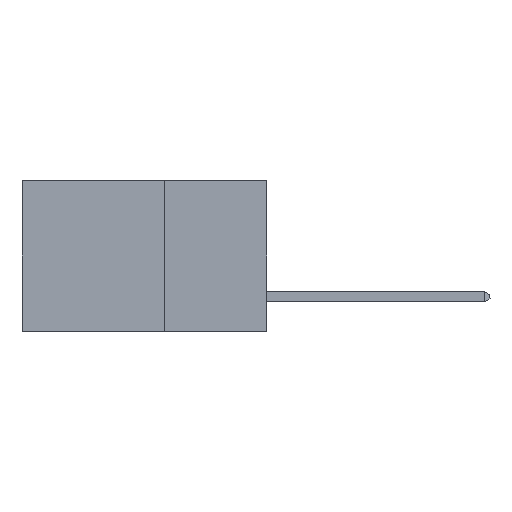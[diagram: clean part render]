
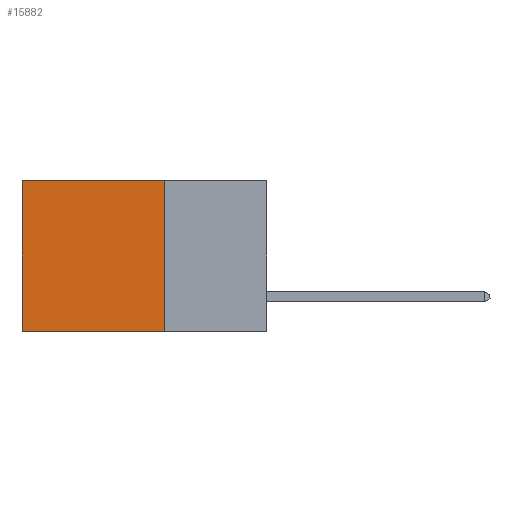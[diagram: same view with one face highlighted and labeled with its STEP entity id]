
A CAD part, left-side view. The second image highlights one B-rep face of the part: STEP entity #15882.
In plain terms, the highlighted planar face has unit normal (-1, 0, 0).
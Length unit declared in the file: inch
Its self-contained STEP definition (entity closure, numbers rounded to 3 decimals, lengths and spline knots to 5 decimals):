
#60 = CARTESIAN_POINT ( 'NONE',  ( 0.2875, 0.25, -0.37 ) ) ;
#1473 = LINE ( 'NONE', #2595, #8041 ) ;
#2060 = ORIENTED_EDGE ( 'NONE', *, *, #10140, .T. ) ;
#2313 = CARTESIAN_POINT ( 'NONE',  ( 0.2875, 0.25, 0. ) ) ;
#2595 = CARTESIAN_POINT ( 'NONE',  ( 0.2875, 0.6, 0. ) ) ;
#3277 = VERTEX_POINT ( 'NONE', #14177 ) ;
#4044 = DIRECTION ( 'NONE',  ( 0., 0., -1. ) ) ;
#4295 = PLANE ( 'NONE',  #15680 ) ;
#4554 = VECTOR ( 'NONE', #10521, 39.37008 ) ;
#4685 = VERTEX_POINT ( 'NONE', #15524 ) ;
#4790 = ORIENTED_EDGE ( 'NONE', *, *, #6001, .T. ) ;
#5188 = CARTESIAN_POINT ( 'NONE',  ( 0.2875, 0.25, -0.37 ) ) ;
#5407 = LINE ( 'NONE', #2313, #4554 ) ;
#6001 = EDGE_CURVE ( 'NONE', #12307, #3277, #5407, .T. ) ;
#6719 = FACE_OUTER_BOUND ( 'NONE', #9423, .T. ) ;
#7062 = DIRECTION ( 'NONE',  ( 0., 0., -1. ) ) ;
#7885 = ORIENTED_EDGE ( 'NONE', *, *, #8242, .F. ) ;
#7898 = EDGE_CURVE ( 'NONE', #12307, #12580, #13830, .T. ) ;
#8041 = VECTOR ( 'NONE', #4044, 39.37008 ) ;
#8242 = EDGE_CURVE ( 'NONE', #12580, #4685, #14992, .T. ) ;
#8834 = CARTESIAN_POINT ( 'NONE',  ( 0.2875, 0.25, 0. ) ) ;
#9423 = EDGE_LOOP ( 'NONE', ( #2060, #7885, #16205, #4790 ) ) ;
#10140 = EDGE_CURVE ( 'NONE', #3277, #4685, #1473, .T. ) ;
#10419 = VECTOR ( 'NONE', #10438, 39.37008 ) ;
#10438 = DIRECTION ( 'NONE',  ( 0., 0., -1. ) ) ;
#10521 = DIRECTION ( 'NONE',  ( 0., 1., 0. ) ) ;
#11008 = CARTESIAN_POINT ( 'NONE',  ( 0.2875, 0.25, 0. ) ) ;
#11138 = DIRECTION ( 'NONE',  ( 0., 1., 0. ) ) ;
#11599 = VECTOR ( 'NONE', #11138, 39.37008 ) ;
#12307 = VERTEX_POINT ( 'NONE', #8834 ) ;
#12580 = VERTEX_POINT ( 'NONE', #5188 ) ;
#13830 = LINE ( 'NONE', #15503, #10419 ) ;
#14177 = CARTESIAN_POINT ( 'NONE',  ( 0.2875, 0.6, 0. ) ) ;
#14868 = DIRECTION ( 'NONE',  ( 1., 0., 0. ) ) ;
#14992 = LINE ( 'NONE', #60, #11599 ) ;
#15503 = CARTESIAN_POINT ( 'NONE',  ( 0.2875, 0.25, 0. ) ) ;
#15524 = CARTESIAN_POINT ( 'NONE',  ( 0.2875, 0.6, -0.37 ) ) ;
#15680 = AXIS2_PLACEMENT_3D ( 'NONE', #11008, #14868, #7062 ) ;
#15882 = ADVANCED_FACE ( 'NONE', ( #6719 ), #4295, .F. ) ;
#16205 = ORIENTED_EDGE ( 'NONE', *, *, #7898, .F. ) ;
